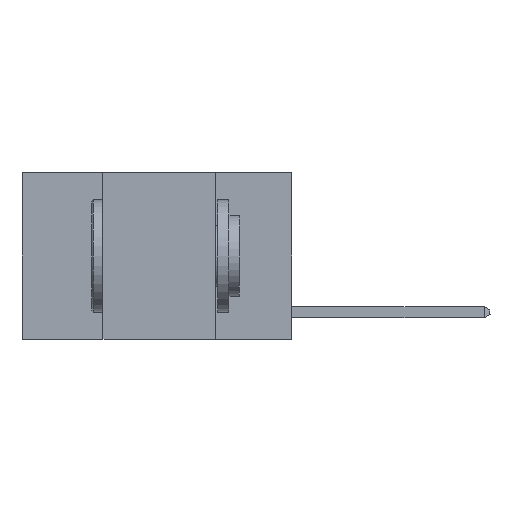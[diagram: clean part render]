
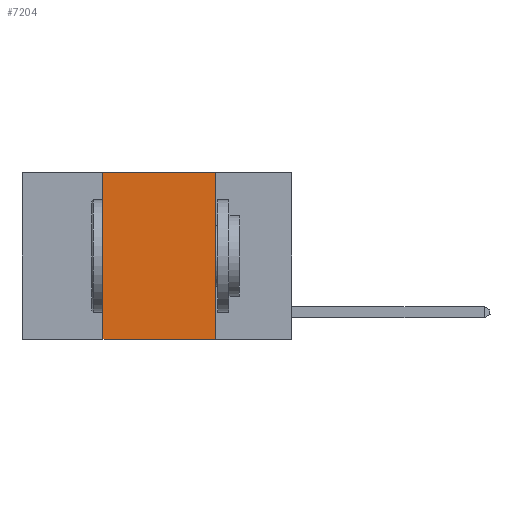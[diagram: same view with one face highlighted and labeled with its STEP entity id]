
A CAD part, left-side view. The second image highlights one B-rep face of the part: STEP entity #7204.
In plain terms, the highlighted planar face has unit normal (-1, 0, 0).
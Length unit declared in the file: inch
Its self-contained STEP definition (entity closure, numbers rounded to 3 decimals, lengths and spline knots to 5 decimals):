
#352 = LINE ( 'NONE', #18613, #12898 ) ;
#367 = EDGE_CURVE ( 'NONE', #6341, #11454, #14211, .T. ) ;
#522 = EDGE_CURVE ( 'NONE', #22598, #11454, #5735, .T. ) ;
#1041 = ORIENTED_EDGE ( 'NONE', *, *, #23858, .F. ) ;
#4575 = FACE_OUTER_BOUND ( 'NONE', #12886, .T. ) ;
#5224 = VECTOR ( 'NONE', #6610, 39.37008 ) ;
#5735 = LINE ( 'NONE', #12755, #23147 ) ;
#5771 = LINE ( 'NONE', #22390, #8908 ) ;
#5879 = VERTEX_POINT ( 'NONE', #21466 ) ;
#6341 = VERTEX_POINT ( 'NONE', #11750 ) ;
#6610 = DIRECTION ( 'NONE',  ( 0., 0., -1. ) ) ;
#7204 = ADVANCED_FACE ( 'NONE', ( #4575 ), #11574, .F. ) ;
#7974 = CARTESIAN_POINT ( 'NONE',  ( 0., 0.6, 0. ) ) ;
#8708 = EDGE_CURVE ( 'NONE', #22598, #5879, #352, .T. ) ;
#8908 = VECTOR ( 'NONE', #9420, 39.37008 ) ;
#9420 = DIRECTION ( 'NONE',  ( 0., -1., 0. ) ) ;
#9498 = DIRECTION ( 'NONE',  ( 0., -1., 0. ) ) ;
#9515 = DIRECTION ( 'NONE',  ( 0., 0., 1. ) ) ;
#10126 = ORIENTED_EDGE ( 'NONE', *, *, #8708, .F. ) ;
#10591 = CARTESIAN_POINT ( 'NONE',  ( 0., 0.17, 0. ) ) ;
#11454 = VERTEX_POINT ( 'NONE', #15150 ) ;
#11574 = PLANE ( 'NONE',  #19770 ) ;
#11750 = CARTESIAN_POINT ( 'NONE',  ( 0., 0.17, 0. ) ) ;
#12755 = CARTESIAN_POINT ( 'NONE',  ( 0., 0.6, -0.37 ) ) ;
#12886 = EDGE_LOOP ( 'NONE', ( #20166, #1041, #10126, #19940 ) ) ;
#12898 = VECTOR ( 'NONE', #9515, 39.37008 ) ;
#13116 = CARTESIAN_POINT ( 'NONE',  ( 0., 0.42, -0.37 ) ) ;
#14211 = LINE ( 'NONE', #10591, #5224 ) ;
#15150 = CARTESIAN_POINT ( 'NONE',  ( 0., 0.17, -0.37 ) ) ;
#18613 = CARTESIAN_POINT ( 'NONE',  ( 0., 0.42, 0. ) ) ;
#19770 = AXIS2_PLACEMENT_3D ( 'NONE', #7974, #20929, #22747 ) ;
#19940 = ORIENTED_EDGE ( 'NONE', *, *, #522, .T. ) ;
#20166 = ORIENTED_EDGE ( 'NONE', *, *, #367, .F. ) ;
#20929 = DIRECTION ( 'NONE',  ( 1., 0., 0. ) ) ;
#21466 = CARTESIAN_POINT ( 'NONE',  ( 0., 0.42, 0. ) ) ;
#22390 = CARTESIAN_POINT ( 'NONE',  ( 0., 0.6, 0. ) ) ;
#22598 = VERTEX_POINT ( 'NONE', #13116 ) ;
#22747 = DIRECTION ( 'NONE',  ( 0., 0., -1. ) ) ;
#23147 = VECTOR ( 'NONE', #9498, 39.37008 ) ;
#23858 = EDGE_CURVE ( 'NONE', #5879, #6341, #5771, .T. ) ;
